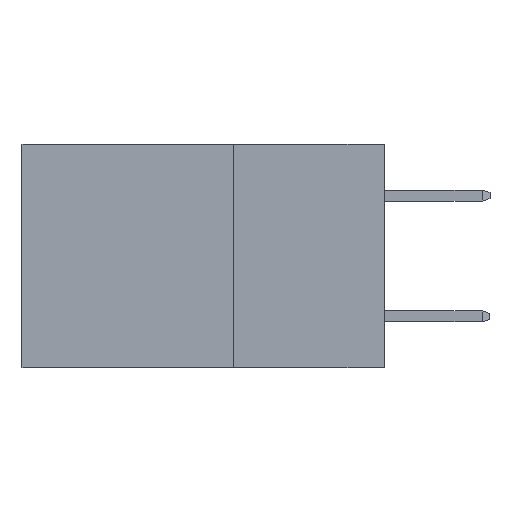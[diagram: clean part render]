
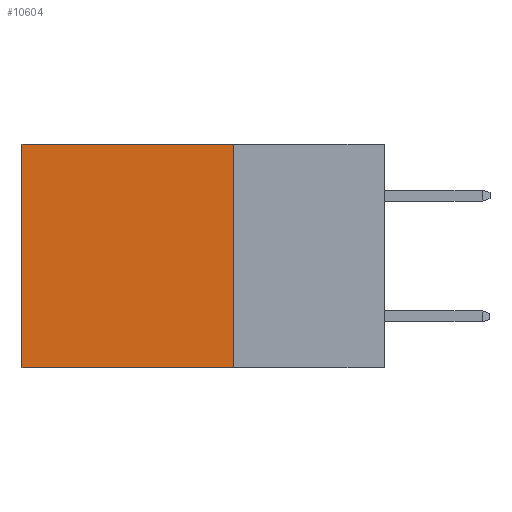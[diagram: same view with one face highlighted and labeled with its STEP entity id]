
A CAD part, left-side view. The second image highlights one B-rep face of the part: STEP entity #10604.
In plain terms, the highlighted planar face has unit normal (-1, 0, 0).
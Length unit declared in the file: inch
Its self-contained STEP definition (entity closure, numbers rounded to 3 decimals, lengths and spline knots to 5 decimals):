
#500 = PLANE ( 'NONE',  #12688 ) ;
#540 = ORIENTED_EDGE ( 'NONE', *, *, #3611, .T. ) ;
#2823 = CARTESIAN_POINT ( 'NONE',  ( 0.298, 0.6, 0. ) ) ;
#3575 = VERTEX_POINT ( 'NONE', #11260 ) ;
#3611 = EDGE_CURVE ( 'NONE', #7731, #4357, #10273, .T. ) ;
#3783 = ORIENTED_EDGE ( 'NONE', *, *, #5143, .F. ) ;
#4339 = VECTOR ( 'NONE', #6139, 39.37008 ) ;
#4357 = VERTEX_POINT ( 'NONE', #2823 ) ;
#4891 = VECTOR ( 'NONE', #5902, 39.37008 ) ;
#5027 = EDGE_CURVE ( 'NONE', #3575, #6623, #12018, .T. ) ;
#5080 = CARTESIAN_POINT ( 'NONE',  ( 0.298, 0.25, 0. ) ) ;
#5143 = EDGE_CURVE ( 'NONE', #7731, #3575, #12812, .T. ) ;
#5814 = DIRECTION ( 'NONE',  ( 1., 0., 0. ) ) ;
#5902 = DIRECTION ( 'NONE',  ( 0., 1., 0. ) ) ;
#5934 = EDGE_CURVE ( 'NONE', #4357, #6623, #13465, .T. ) ;
#5965 = CARTESIAN_POINT ( 'NONE',  ( 0.298, 0.25, -0.37 ) ) ;
#6139 = DIRECTION ( 'NONE',  ( 0., 0., -1. ) ) ;
#6623 = VERTEX_POINT ( 'NONE', #11645 ) ;
#7162 = EDGE_LOOP ( 'NONE', ( #9799, #10907, #3783, #540 ) ) ;
#7329 = DIRECTION ( 'NONE',  ( 0., 0., -1. ) ) ;
#7401 = FACE_OUTER_BOUND ( 'NONE', #7162, .T. ) ;
#7731 = VERTEX_POINT ( 'NONE', #11311 ) ;
#8040 = DIRECTION ( 'NONE',  ( 0., 0., -1. ) ) ;
#9147 = CARTESIAN_POINT ( 'NONE',  ( 0.298, 0.25, 0. ) ) ;
#9197 = VECTOR ( 'NONE', #12347, 39.37008 ) ;
#9474 = CARTESIAN_POINT ( 'NONE',  ( 0.298, 0.6, 0. ) ) ;
#9799 = ORIENTED_EDGE ( 'NONE', *, *, #5934, .T. ) ;
#10273 = LINE ( 'NONE', #9147, #4891 ) ;
#10604 = ADVANCED_FACE ( 'NONE', ( #7401 ), #500, .F. ) ;
#10907 = ORIENTED_EDGE ( 'NONE', *, *, #5027, .F. ) ;
#11260 = CARTESIAN_POINT ( 'NONE',  ( 0.298, 0.25, -0.37 ) ) ;
#11311 = CARTESIAN_POINT ( 'NONE',  ( 0.298, 0.25, 0. ) ) ;
#11645 = CARTESIAN_POINT ( 'NONE',  ( 0.298, 0.6, -0.37 ) ) ;
#12018 = LINE ( 'NONE', #5965, #9197 ) ;
#12347 = DIRECTION ( 'NONE',  ( 0., 1., 0. ) ) ;
#12688 = AXIS2_PLACEMENT_3D ( 'NONE', #13289, #5814, #8040 ) ;
#12812 = LINE ( 'NONE', #5080, #4339 ) ;
#12815 = VECTOR ( 'NONE', #7329, 39.37008 ) ;
#13289 = CARTESIAN_POINT ( 'NONE',  ( 0.298, 0.25, 0. ) ) ;
#13465 = LINE ( 'NONE', #9474, #12815 ) ;
